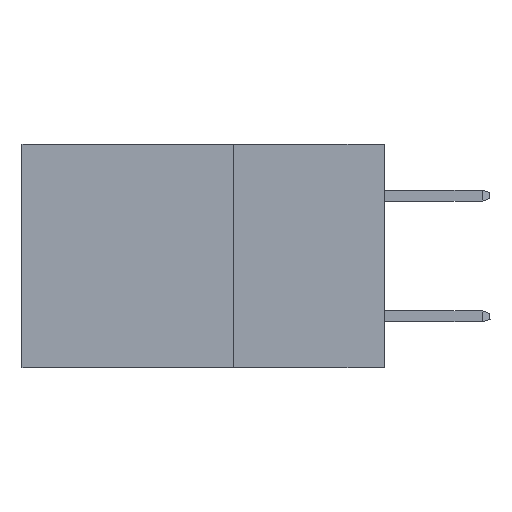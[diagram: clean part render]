
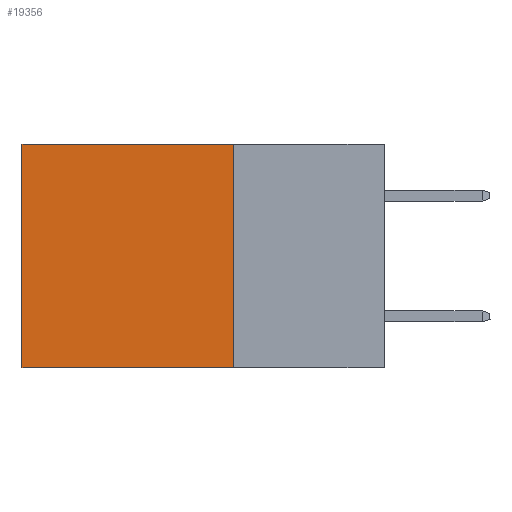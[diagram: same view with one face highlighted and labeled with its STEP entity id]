
A CAD part, left-side view. The second image highlights one B-rep face of the part: STEP entity #19356.
In plain terms, the highlighted planar face has unit normal (-1, 0, 0).
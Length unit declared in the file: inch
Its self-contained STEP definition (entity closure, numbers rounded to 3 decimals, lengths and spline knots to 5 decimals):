
#106 = ORIENTED_EDGE ( 'NONE', *, *, #14305, .F. ) ;
#195 = CARTESIAN_POINT ( 'NONE',  ( 0.298, 0.25, 0. ) ) ;
#713 = EDGE_CURVE ( 'NONE', #25723, #23900, #15462, .T. ) ;
#2950 = DIRECTION ( 'NONE',  ( 0., 1., 0. ) ) ;
#3391 = DIRECTION ( 'NONE',  ( 0., 0., -1. ) ) ;
#5569 = ORIENTED_EDGE ( 'NONE', *, *, #19534, .T. ) ;
#5595 = CARTESIAN_POINT ( 'NONE',  ( 0.298, 0.25, 0. ) ) ;
#8081 = CARTESIAN_POINT ( 'NONE',  ( 0.298, 0.25, 0. ) ) ;
#8532 = VERTEX_POINT ( 'NONE', #8081 ) ;
#9297 = CARTESIAN_POINT ( 'NONE',  ( 0.298, 0.25, -0.37 ) ) ;
#9463 = DIRECTION ( 'NONE',  ( 0., 0., -1. ) ) ;
#9902 = CARTESIAN_POINT ( 'NONE',  ( 0.298, 0.25, -0.37 ) ) ;
#10835 = LINE ( 'NONE', #9902, #29336 ) ;
#11063 = CARTESIAN_POINT ( 'NONE',  ( 0.298, 0.25, 0. ) ) ;
#11873 = CARTESIAN_POINT ( 'NONE',  ( 0.298, 0.6, -0.37 ) ) ;
#12056 = AXIS2_PLACEMENT_3D ( 'NONE', #5595, #12657, #3391 ) ;
#12314 = DIRECTION ( 'NONE',  ( 0., 0., -1. ) ) ;
#12657 = DIRECTION ( 'NONE',  ( 1., 0., 0. ) ) ;
#13582 = LINE ( 'NONE', #11063, #27544 ) ;
#14304 = ORIENTED_EDGE ( 'NONE', *, *, #29462, .F. ) ;
#14305 = EDGE_CURVE ( 'NONE', #8532, #23192, #23777, .T. ) ;
#14706 = VECTOR ( 'NONE', #9463, 39.37008 ) ;
#15194 = PLANE ( 'NONE',  #12056 ) ;
#15462 = LINE ( 'NONE', #24310, #14706 ) ;
#16042 = CARTESIAN_POINT ( 'NONE',  ( 0.298, 0.6, 0. ) ) ;
#16877 = EDGE_LOOP ( 'NONE', ( #20516, #14304, #106, #5569 ) ) ;
#18548 = VECTOR ( 'NONE', #12314, 39.37008 ) ;
#18794 = DIRECTION ( 'NONE',  ( 0., 1., 0. ) ) ;
#19356 = ADVANCED_FACE ( 'NONE', ( #21191 ), #15194, .F. ) ;
#19534 = EDGE_CURVE ( 'NONE', #8532, #25723, #13582, .T. ) ;
#20516 = ORIENTED_EDGE ( 'NONE', *, *, #713, .T. ) ;
#21191 = FACE_OUTER_BOUND ( 'NONE', #16877, .T. ) ;
#23192 = VERTEX_POINT ( 'NONE', #9297 ) ;
#23777 = LINE ( 'NONE', #195, #18548 ) ;
#23900 = VERTEX_POINT ( 'NONE', #11873 ) ;
#24310 = CARTESIAN_POINT ( 'NONE',  ( 0.298, 0.6, 0. ) ) ;
#25723 = VERTEX_POINT ( 'NONE', #16042 ) ;
#27544 = VECTOR ( 'NONE', #18794, 39.37008 ) ;
#29336 = VECTOR ( 'NONE', #2950, 39.37008 ) ;
#29462 = EDGE_CURVE ( 'NONE', #23192, #23900, #10835, .T. ) ;
